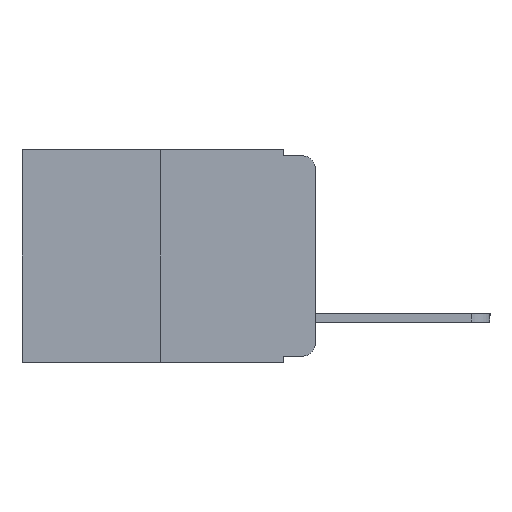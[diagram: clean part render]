
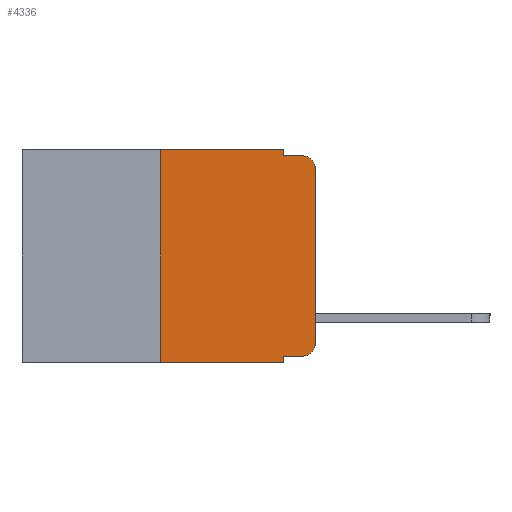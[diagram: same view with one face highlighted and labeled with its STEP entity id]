
A CAD part, left-side view. The second image highlights one B-rep face of the part: STEP entity #4336.
In plain terms, the highlighted planar face has unit normal (-1, 0, 0).
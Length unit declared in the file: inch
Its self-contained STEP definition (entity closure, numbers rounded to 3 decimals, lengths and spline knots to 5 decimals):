
#5 = EDGE_CURVE ( 'NONE', #6710, #542, #11342, .T. ) ;
#292 = VERTEX_POINT ( 'NONE', #5285 ) ;
#522 = ORIENTED_EDGE ( 'NONE', *, *, #6356, .F. ) ;
#542 = VERTEX_POINT ( 'NONE', #3523 ) ;
#601 = AXIS2_PLACEMENT_3D ( 'NONE', #6071, #10727, #5076 ) ;
#828 = EDGE_CURVE ( 'NONE', #4396, #8338, #5534, .T. ) ;
#884 = EDGE_CURVE ( 'NONE', #2928, #5856, #12232, .T. ) ;
#962 = VERTEX_POINT ( 'NONE', #4243 ) ;
#1388 = VERTEX_POINT ( 'NONE', #2893 ) ;
#1662 = LINE ( 'NONE', #3750, #10874 ) ;
#1767 = CARTESIAN_POINT ( 'NONE',  ( 0., 0.02, -0.03 ) ) ;
#1863 = PLANE ( 'NONE',  #601 ) ;
#2006 = CARTESIAN_POINT ( 'NONE',  ( 0., 0., -0.03 ) ) ;
#2009 = CARTESIAN_POINT ( 'NONE',  ( 0., 0.02, -0.313 ) ) ;
#2266 = VECTOR ( 'NONE', #2657, 39.37008 ) ;
#2530 = CARTESIAN_POINT ( 'NONE',  ( 0., 0.25, -0.343 ) ) ;
#2657 = DIRECTION ( 'NONE',  ( 0., 0., -1. ) ) ;
#2893 = CARTESIAN_POINT ( 'NONE',  ( 0., 0.051, -0.333 ) ) ;
#2928 = VERTEX_POINT ( 'NONE', #9375 ) ;
#3168 = CARTESIAN_POINT ( 'NONE',  ( 0., 0.25, 0. ) ) ;
#3523 = CARTESIAN_POINT ( 'NONE',  ( 0., 0.25, 0. ) ) ;
#3716 = ORIENTED_EDGE ( 'NONE', *, *, #884, .T. ) ;
#3750 = CARTESIAN_POINT ( 'NONE',  ( 0., 0.051, 0. ) ) ;
#3885 = CARTESIAN_POINT ( 'NONE',  ( 0., 0.051, -0.01 ) ) ;
#4243 = CARTESIAN_POINT ( 'NONE',  ( 0., 0.051, -0.343 ) ) ;
#4293 = DIRECTION ( 'NONE',  ( 0., 0., 1. ) ) ;
#4324 = VECTOR ( 'NONE', #4293, 39.37008 ) ;
#4336 = ADVANCED_FACE ( 'NONE', ( #5303 ), #1863, .F. ) ;
#4396 = VERTEX_POINT ( 'NONE', #2006 ) ;
#4718 = ORIENTED_EDGE ( 'NONE', *, *, #828, .T. ) ;
#4825 = DIRECTION ( 'NONE',  ( 0., -1., 0. ) ) ;
#5076 = DIRECTION ( 'NONE',  ( 0., 0., -1. ) ) ;
#5154 = EDGE_CURVE ( 'NONE', #292, #8338, #6883, .T. ) ;
#5285 = CARTESIAN_POINT ( 'NONE',  ( 0., 0.051, -0.01 ) ) ;
#5303 = FACE_OUTER_BOUND ( 'NONE', #9737, .T. ) ;
#5323 = EDGE_CURVE ( 'NONE', #5856, #4396, #7679, .T. ) ;
#5534 = CIRCLE ( 'NONE', #5804, 0.02 ) ;
#5570 = CARTESIAN_POINT ( 'NONE',  ( 0., 0., -0.313 ) ) ;
#5635 = DIRECTION ( 'NONE',  ( 0., 0., 1. ) ) ;
#5804 = AXIS2_PLACEMENT_3D ( 'NONE', #1767, #7042, #8440 ) ;
#5827 = ORIENTED_EDGE ( 'NONE', *, *, #5, .F. ) ;
#5842 = EDGE_CURVE ( 'NONE', #1388, #2928, #9617, .T. ) ;
#5856 = VERTEX_POINT ( 'NONE', #5570 ) ;
#5969 = DIRECTION ( 'NONE',  ( 0., -1., 0. ) ) ;
#6071 = CARTESIAN_POINT ( 'NONE',  ( 0., 0.473, 0. ) ) ;
#6132 = ORIENTED_EDGE ( 'NONE', *, *, #5842, .T. ) ;
#6356 = EDGE_CURVE ( 'NONE', #1388, #962, #1662, .T. ) ;
#6494 = DIRECTION ( 'NONE',  ( 0., -1., 0. ) ) ;
#6559 = VECTOR ( 'NONE', #5969, 39.37008 ) ;
#6710 = VERTEX_POINT ( 'NONE', #2530 ) ;
#6836 = CARTESIAN_POINT ( 'NONE',  ( 0., 0.051, 0. ) ) ;
#6854 = VECTOR ( 'NONE', #6494, 39.37008 ) ;
#6883 = LINE ( 'NONE', #3885, #6559 ) ;
#7042 = DIRECTION ( 'NONE',  ( -1., 0., 0. ) ) ;
#7080 = EDGE_CURVE ( 'NONE', #9572, #292, #8099, .T. ) ;
#7100 = ORIENTED_EDGE ( 'NONE', *, *, #5323, .T. ) ;
#7116 = CARTESIAN_POINT ( 'NONE',  ( 0., 0.473, 0. ) ) ;
#7160 = AXIS2_PLACEMENT_3D ( 'NONE', #2009, #9096, #8194 ) ;
#7421 = ORIENTED_EDGE ( 'NONE', *, *, #5154, .F. ) ;
#7679 = LINE ( 'NONE', #10036, #4324 ) ;
#7744 = ORIENTED_EDGE ( 'NONE', *, *, #7080, .F. ) ;
#8094 = DIRECTION ( 'NONE',  ( 0., -1., 0. ) ) ;
#8099 = LINE ( 'NONE', #12168, #2266 ) ;
#8194 = DIRECTION ( 'NONE',  ( 0., 0., -1. ) ) ;
#8338 = VERTEX_POINT ( 'NONE', #11767 ) ;
#8418 = ORIENTED_EDGE ( 'NONE', *, *, #12295, .T. ) ;
#8440 = DIRECTION ( 'NONE',  ( 0., 0., -1. ) ) ;
#8977 = EDGE_CURVE ( 'NONE', #542, #9572, #9423, .T. ) ;
#9047 = VECTOR ( 'NONE', #5635, 39.37008 ) ;
#9096 = DIRECTION ( 'NONE',  ( -1., 0., 0. ) ) ;
#9375 = CARTESIAN_POINT ( 'NONE',  ( 0., 0.02, -0.333 ) ) ;
#9423 = LINE ( 'NONE', #7116, #11705 ) ;
#9572 = VERTEX_POINT ( 'NONE', #6836 ) ;
#9617 = LINE ( 'NONE', #10203, #6854 ) ;
#9737 = EDGE_LOOP ( 'NONE', ( #7100, #4718, #7421, #7744, #12333, #5827, #8418, #522, #6132, #3716 ) ) ;
#10036 = CARTESIAN_POINT ( 'NONE',  ( 0., 0., 0. ) ) ;
#10203 = CARTESIAN_POINT ( 'NONE',  ( 0., 0.051, -0.333 ) ) ;
#10727 = DIRECTION ( 'NONE',  ( 1., 0., 0. ) ) ;
#10874 = VECTOR ( 'NONE', #11337, 39.37008 ) ;
#11337 = DIRECTION ( 'NONE',  ( 0., 0., -1. ) ) ;
#11342 = LINE ( 'NONE', #3168, #9047 ) ;
#11373 = VECTOR ( 'NONE', #4825, 39.37008 ) ;
#11639 = LINE ( 'NONE', #12155, #11373 ) ;
#11705 = VECTOR ( 'NONE', #8094, 39.37008 ) ;
#11767 = CARTESIAN_POINT ( 'NONE',  ( 0., 0.02, -0.01 ) ) ;
#12155 = CARTESIAN_POINT ( 'NONE',  ( 0., 0.473, -0.343 ) ) ;
#12168 = CARTESIAN_POINT ( 'NONE',  ( 0., 0.051, 0. ) ) ;
#12232 = CIRCLE ( 'NONE', #7160, 0.02 ) ;
#12295 = EDGE_CURVE ( 'NONE', #6710, #962, #11639, .T. ) ;
#12333 = ORIENTED_EDGE ( 'NONE', *, *, #8977, .F. ) ;
